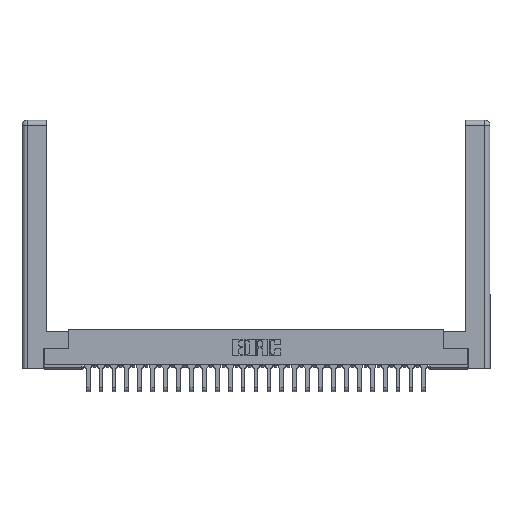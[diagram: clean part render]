
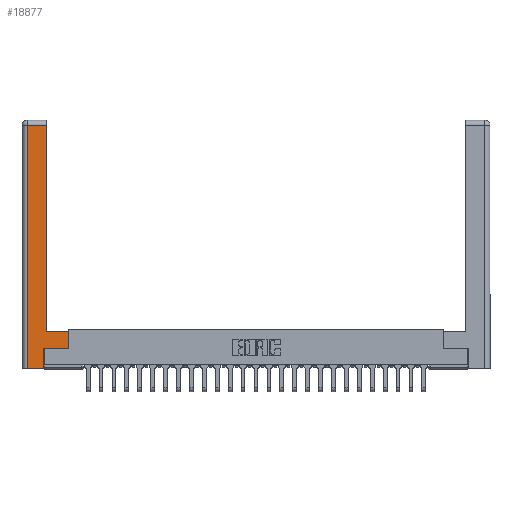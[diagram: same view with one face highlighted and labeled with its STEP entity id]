
A CAD part, top view. The second image highlights one B-rep face of the part: STEP entity #18877.
In plain terms, the highlighted planar face has unit normal (0, 0, 1).
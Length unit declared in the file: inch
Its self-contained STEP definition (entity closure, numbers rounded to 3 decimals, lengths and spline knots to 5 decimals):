
#264 = CARTESIAN_POINT ( 'NONE',  ( 0.265, 0., 0. ) ) ;
#349 = CARTESIAN_POINT ( 'NONE',  ( 0.295, 0.45, 0. ) ) ;
#1403 = LINE ( 'NONE', #29633, #24098 ) ;
#2793 = DIRECTION ( 'NONE',  ( 0., 0., -1. ) ) ;
#3077 = CARTESIAN_POINT ( 'NONE',  ( 0.295, 3., 0. ) ) ;
#3092 = LINE ( 'NONE', #15209, #11366 ) ;
#3148 = VERTEX_POINT ( 'NONE', #8148 ) ;
#3488 = EDGE_CURVE ( 'NONE', #20148, #17376, #3092, .T. ) ;
#3494 = VECTOR ( 'NONE', #3775, 39.37008 ) ;
#3680 = VECTOR ( 'NONE', #3996, 39.37008 ) ;
#3775 = DIRECTION ( 'NONE',  ( -1., 0., 0. ) ) ;
#3996 = DIRECTION ( 'NONE',  ( 0., 1., 0. ) ) ;
#4783 = CARTESIAN_POINT ( 'NONE',  ( 0.295, 0.45, 0. ) ) ;
#4842 = ORIENTED_EDGE ( 'NONE', *, *, #3488, .T. ) ;
#5041 = VERTEX_POINT ( 'NONE', #6632 ) ;
#6632 = CARTESIAN_POINT ( 'NONE',  ( 0.0615, 2.94, 0. ) ) ;
#7147 = EDGE_LOOP ( 'NONE', ( #11689, #26729, #22060, #11006, #9040, #4842, #7840, #18071 ) ) ;
#7160 = VECTOR ( 'NONE', #18222, 39.37008 ) ;
#7185 = DIRECTION ( 'NONE',  ( 0., 1., 0. ) ) ;
#7840 = ORIENTED_EDGE ( 'NONE', *, *, #21128, .T. ) ;
#8148 = CARTESIAN_POINT ( 'NONE',  ( 0.565, 0.45, 0. ) ) ;
#8350 = VERTEX_POINT ( 'NONE', #23302 ) ;
#8517 = CARTESIAN_POINT ( 'NONE',  ( 0.265, 0.245, 0. ) ) ;
#9040 = ORIENTED_EDGE ( 'NONE', *, *, #27048, .T. ) ;
#9600 = FACE_OUTER_BOUND ( 'NONE', #7147, .T. ) ;
#10177 = LINE ( 'NONE', #3077, #23875 ) ;
#10399 = LINE ( 'NONE', #15556, #3494 ) ;
#10476 = LINE ( 'NONE', #8517, #3680 ) ;
#10633 = DIRECTION ( 'NONE',  ( 0., -1., 0. ) ) ;
#10758 = EDGE_CURVE ( 'NONE', #15418, #5041, #10399, .T. ) ;
#11006 = ORIENTED_EDGE ( 'NONE', *, *, #29579, .T. ) ;
#11366 = VECTOR ( 'NONE', #19192, 39.37008 ) ;
#11689 = ORIENTED_EDGE ( 'NONE', *, *, #14258, .T. ) ;
#14258 = EDGE_CURVE ( 'NONE', #24395, #15418, #10177, .T. ) ;
#15209 = CARTESIAN_POINT ( 'NONE',  ( 0.565, 0.245, 0. ) ) ;
#15418 = VERTEX_POINT ( 'NONE', #19800 ) ;
#15556 = CARTESIAN_POINT ( 'NONE',  ( 0.0615, 2.94, 0. ) ) ;
#15751 = EDGE_CURVE ( 'NONE', #3148, #24395, #16839, .T. ) ;
#16839 = LINE ( 'NONE', #349, #28791 ) ;
#17376 = VERTEX_POINT ( 'NONE', #25641 ) ;
#17698 = CARTESIAN_POINT ( 'NONE',  ( 0.265, 0.245, 0. ) ) ;
#17758 = VECTOR ( 'NONE', #28320, 39.37008 ) ;
#18071 = ORIENTED_EDGE ( 'NONE', *, *, #15751, .T. ) ;
#18222 = DIRECTION ( 'NONE',  ( 0., 1., 0. ) ) ;
#18577 = CARTESIAN_POINT ( 'NONE',  ( 0., 0., 0. ) ) ;
#18877 = ADVANCED_FACE ( 'NONE', ( #9600 ), #21171, .F. ) ;
#19192 = DIRECTION ( 'NONE',  ( 1., 0., 0. ) ) ;
#19314 = CARTESIAN_POINT ( 'NONE',  ( 0.0615, 0., 0. ) ) ;
#19800 = CARTESIAN_POINT ( 'NONE',  ( 0.295, 2.94, 0. ) ) ;
#20148 = VERTEX_POINT ( 'NONE', #17698 ) ;
#20818 = LINE ( 'NONE', #23232, #7160 ) ;
#21128 = EDGE_CURVE ( 'NONE', #17376, #3148, #20818, .T. ) ;
#21171 = PLANE ( 'NONE',  #23509 ) ;
#22060 = ORIENTED_EDGE ( 'NONE', *, *, #22328, .T. ) ;
#22112 = VERTEX_POINT ( 'NONE', #19314 ) ;
#22328 = EDGE_CURVE ( 'NONE', #5041, #22112, #1403, .T. ) ;
#23232 = CARTESIAN_POINT ( 'NONE',  ( 0.565, 0.45, 0. ) ) ;
#23302 = CARTESIAN_POINT ( 'NONE',  ( 0.265, 0., 0. ) ) ;
#23389 = DIRECTION ( 'NONE',  ( -1., 0., 0. ) ) ;
#23509 = AXIS2_PLACEMENT_3D ( 'NONE', #18577, #2793, #27714 ) ;
#23875 = VECTOR ( 'NONE', #7185, 39.37008 ) ;
#24098 = VECTOR ( 'NONE', #10633, 39.37008 ) ;
#24395 = VERTEX_POINT ( 'NONE', #4783 ) ;
#25641 = CARTESIAN_POINT ( 'NONE',  ( 0.565, 0.245, 0. ) ) ;
#26729 = ORIENTED_EDGE ( 'NONE', *, *, #10758, .T. ) ;
#27048 = EDGE_CURVE ( 'NONE', #8350, #20148, #10476, .T. ) ;
#27714 = DIRECTION ( 'NONE',  ( -1., 0., 0. ) ) ;
#28035 = LINE ( 'NONE', #264, #17758 ) ;
#28320 = DIRECTION ( 'NONE',  ( 1., 0., 0. ) ) ;
#28791 = VECTOR ( 'NONE', #23389, 39.37008 ) ;
#29579 = EDGE_CURVE ( 'NONE', #22112, #8350, #28035, .T. ) ;
#29633 = CARTESIAN_POINT ( 'NONE',  ( 0.0615, 0., 0. ) ) ;
